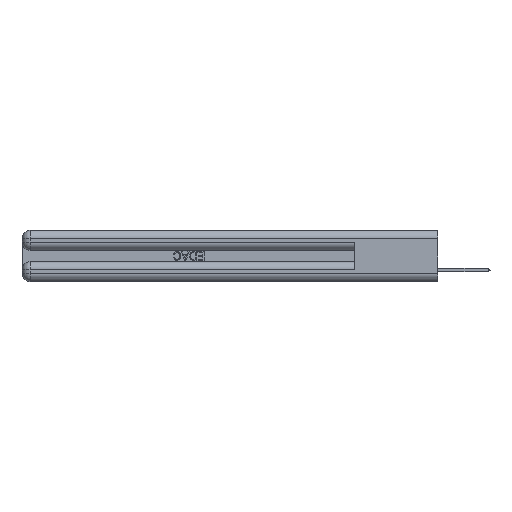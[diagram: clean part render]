
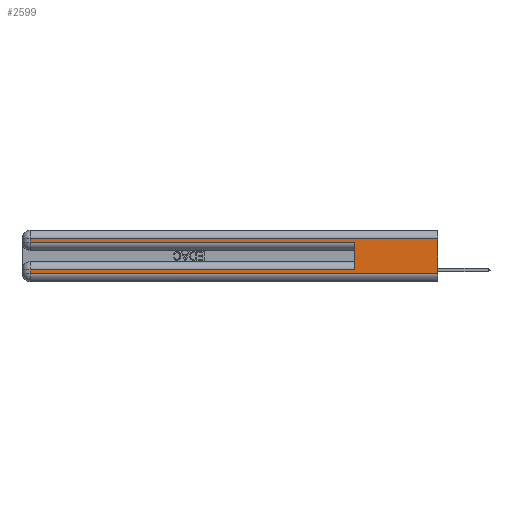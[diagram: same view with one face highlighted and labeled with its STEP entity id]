
A CAD part, left-side view. The second image highlights one B-rep face of the part: STEP entity #2599.
In plain terms, the highlighted planar face has unit normal (-1, 0, 0).
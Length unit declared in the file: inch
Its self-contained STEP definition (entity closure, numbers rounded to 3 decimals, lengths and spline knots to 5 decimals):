
#139 = ORIENTED_EDGE ( 'NONE', *, *, #3167, .T. ) ;
#1487 = ORIENTED_EDGE ( 'NONE', *, *, #21279, .T. ) ;
#2599 = ADVANCED_FACE ( 'NONE', ( #16784 ), #13131, .F. ) ;
#3137 = LINE ( 'NONE', #17272, #19886 ) ;
#3167 = EDGE_CURVE ( 'NONE', #31931, #22905, #31689, .T. ) ;
#3444 = CARTESIAN_POINT ( 'NONE',  ( 0., 2.94, 0.085 ) ) ;
#5051 = DIRECTION ( 'NONE',  ( 0., -1., 0. ) ) ;
#5823 = VERTEX_POINT ( 'NONE', #6203 ) ;
#6203 = CARTESIAN_POINT ( 'NONE',  ( 0., 0.6, 0.285 ) ) ;
#6848 = VECTOR ( 'NONE', #37489, 39.37008 ) ;
#7089 = DIRECTION ( 'NONE',  ( 0., -1., 0. ) ) ;
#7324 = CARTESIAN_POINT ( 'NONE',  ( 0., 2.94, 0.37 ) ) ;
#8267 = LINE ( 'NONE', #9857, #6848 ) ;
#8655 = CARTESIAN_POINT ( 'NONE',  ( 0., 2.94, 0.31 ) ) ;
#9298 = EDGE_CURVE ( 'NONE', #15667, #13713, #3137, .T. ) ;
#9857 = CARTESIAN_POINT ( 'NONE',  ( 0., 2.94, 0.37 ) ) ;
#11121 = DIRECTION ( 'NONE',  ( 0., 1., 0. ) ) ;
#11296 = LINE ( 'NONE', #27973, #38293 ) ;
#12786 = LINE ( 'NONE', #33291, #28166 ) ;
#12988 = CARTESIAN_POINT ( 'NONE',  ( 0., 0., 0.06 ) ) ;
#13131 = PLANE ( 'NONE',  #33137 ) ;
#13211 = VERTEX_POINT ( 'NONE', #39673 ) ;
#13713 = VERTEX_POINT ( 'NONE', #8655 ) ;
#14059 = EDGE_CURVE ( 'NONE', #22326, #5823, #12786, .T. ) ;
#14115 = CARTESIAN_POINT ( 'NONE',  ( 0., 0., 0.06 ) ) ;
#15321 = CARTESIAN_POINT ( 'NONE',  ( 0., 0.6, 0.085 ) ) ;
#15667 = VERTEX_POINT ( 'NONE', #29694 ) ;
#16036 = EDGE_CURVE ( 'NONE', #13211, #22019, #20741, .T. ) ;
#16415 = VECTOR ( 'NONE', #7089, 39.37008 ) ;
#16784 = FACE_OUTER_BOUND ( 'NONE', #16974, .T. ) ;
#16974 = EDGE_LOOP ( 'NONE', ( #32449, #17053, #24764, #34711, #20267, #139, #1487, #34813 ) ) ;
#17053 = ORIENTED_EDGE ( 'NONE', *, *, #9298, .T. ) ;
#17272 = CARTESIAN_POINT ( 'NONE',  ( 0., 0., 0.31 ) ) ;
#17445 = LINE ( 'NONE', #7324, #37264 ) ;
#18453 = EDGE_CURVE ( 'NONE', #31931, #5823, #20105, .T. ) ;
#19886 = VECTOR ( 'NONE', #11121, 39.37008 ) ;
#20105 = LINE ( 'NONE', #38395, #35636 ) ;
#20267 = ORIENTED_EDGE ( 'NONE', *, *, #18453, .F. ) ;
#20741 = LINE ( 'NONE', #12988, #16415 ) ;
#21279 = EDGE_CURVE ( 'NONE', #22905, #13211, #17445, .T. ) ;
#21359 = DIRECTION ( 'NONE',  ( 0., 0., -1. ) ) ;
#21743 = EDGE_CURVE ( 'NONE', #13713, #22326, #8267, .T. ) ;
#22019 = VERTEX_POINT ( 'NONE', #14115 ) ;
#22242 = DIRECTION ( 'NONE',  ( 0., 0., -1. ) ) ;
#22326 = VERTEX_POINT ( 'NONE', #31733 ) ;
#22905 = VERTEX_POINT ( 'NONE', #3444 ) ;
#24764 = ORIENTED_EDGE ( 'NONE', *, *, #21743, .T. ) ;
#26088 = DIRECTION ( 'NONE',  ( 0., 0., 1. ) ) ;
#26137 = DIRECTION ( 'NONE',  ( 0., 0., -1. ) ) ;
#27593 = CARTESIAN_POINT ( 'NONE',  ( 0., 0., 0.085 ) ) ;
#27973 = CARTESIAN_POINT ( 'NONE',  ( 0., 0., 0.37 ) ) ;
#28166 = VECTOR ( 'NONE', #5051, 39.37008 ) ;
#28302 = VECTOR ( 'NONE', #39892, 39.37008 ) ;
#29694 = CARTESIAN_POINT ( 'NONE',  ( 0., 0., 0.31 ) ) ;
#31443 = DIRECTION ( 'NONE',  ( 1., 0., 0. ) ) ;
#31689 = LINE ( 'NONE', #27593, #28302 ) ;
#31733 = CARTESIAN_POINT ( 'NONE',  ( 0., 2.94, 0.285 ) ) ;
#31931 = VERTEX_POINT ( 'NONE', #15321 ) ;
#32449 = ORIENTED_EDGE ( 'NONE', *, *, #36058, .F. ) ;
#33137 = AXIS2_PLACEMENT_3D ( 'NONE', #37423, #31443, #22242 ) ;
#33291 = CARTESIAN_POINT ( 'NONE',  ( 0., 0., 0.285 ) ) ;
#34711 = ORIENTED_EDGE ( 'NONE', *, *, #14059, .T. ) ;
#34813 = ORIENTED_EDGE ( 'NONE', *, *, #16036, .T. ) ;
#35636 = VECTOR ( 'NONE', #26088, 39.37008 ) ;
#36058 = EDGE_CURVE ( 'NONE', #15667, #22019, #11296, .T. ) ;
#37264 = VECTOR ( 'NONE', #26137, 39.37008 ) ;
#37423 = CARTESIAN_POINT ( 'NONE',  ( 0., 0., 0.37 ) ) ;
#37489 = DIRECTION ( 'NONE',  ( 0., 0., -1. ) ) ;
#38293 = VECTOR ( 'NONE', #21359, 39.37008 ) ;
#38395 = CARTESIAN_POINT ( 'NONE',  ( 0., 0.6, 0.145 ) ) ;
#39673 = CARTESIAN_POINT ( 'NONE',  ( 0., 2.94, 0.06 ) ) ;
#39892 = DIRECTION ( 'NONE',  ( 0., 1., 0. ) ) ;
